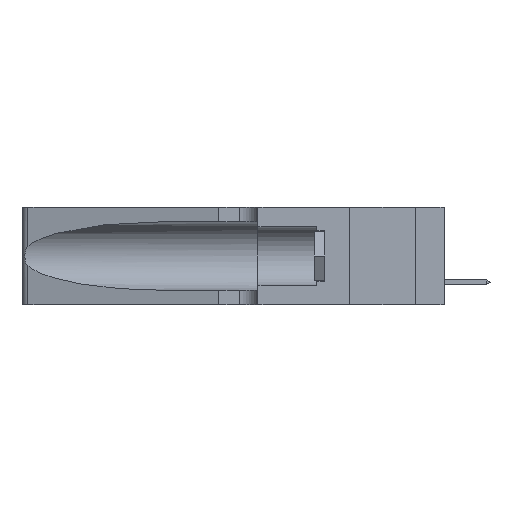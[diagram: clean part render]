
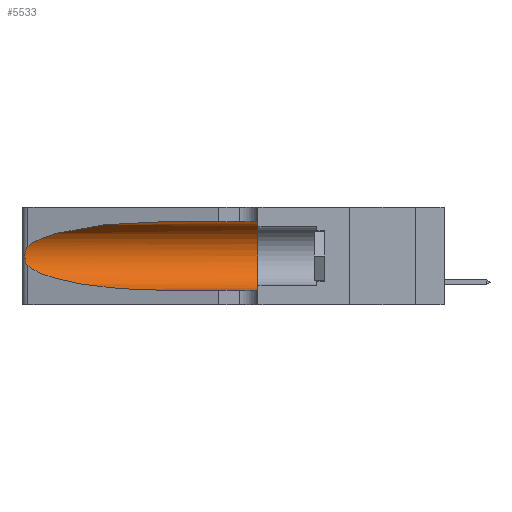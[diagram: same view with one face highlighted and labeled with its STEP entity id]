
A CAD part, left-side view. The second image highlights one B-rep face of the part: STEP entity #5533.
In plain terms, the highlighted cylindrical face has radius 3.308 mm (diameter 6.617 mm), a partial arc.
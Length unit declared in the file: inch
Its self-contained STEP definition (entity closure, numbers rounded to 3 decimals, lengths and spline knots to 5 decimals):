
#84 = CARTESIAN_POINT ( 'NONE',  ( 0.1305, 1.61858, 0.31525 ) ) ;
#409 = CARTESIAN_POINT ( 'NONE',  ( 0.1305, 0.72297, 0.05475 ) ) ;
#952 = CARTESIAN_POINT ( 'NONE',  ( 0.25487, 1.22718, 0.22369 ) ) ;
#1213 = EDGE_LOOP ( 'NONE', ( #17877, #12531, #1446, #14949, #14070, #15062 ) ) ;
#1439 = CARTESIAN_POINT ( 'NONE',  ( 0.25487, 1.22718, 0.14631 ) ) ;
#1446 = ORIENTED_EDGE ( 'NONE', *, *, #3852, .T. ) ;
#1830 = CARTESIAN_POINT ( 'NONE',  ( 0.1305, 1.61858, 0.05475 ) ) ;
#2104 =( BOUNDED_CURVE ( )  B_SPLINE_CURVE ( 3, ( #17723, #7977, #3104, #14460 ),
 .UNSPECIFIED., .F., .F. ) 
 B_SPLINE_CURVE_WITH_KNOTS ( ( 4, 4 ),
 ( 1.5708, 2.84003 ),
 .UNSPECIFIED. ) 
 CURVE ( )  GEOMETRIC_REPRESENTATION_ITEM ( )  RATIONAL_B_SPLINE_CURVE ( ( 1., 0.87, 0.87, 1. ) ) 
 REPRESENTATION_ITEM ( '' )  );
#3032 =( BOUNDED_CURVE ( )  B_SPLINE_CURVE ( 3, ( #16260, #19619, #20978, #14747 ),
 .UNSPECIFIED., .F., .F. ) 
 B_SPLINE_CURVE_WITH_KNOTS ( ( 4, 4 ),
 ( 3.44316, 4.71239 ),
 .UNSPECIFIED. ) 
 CURVE ( )  GEOMETRIC_REPRESENTATION_ITEM ( )  RATIONAL_B_SPLINE_CURVE ( ( 1., 0.87, 0.87, 1. ) ) 
 REPRESENTATION_ITEM ( '' )  );
#3104 = CARTESIAN_POINT ( 'NONE',  ( 0.2373, 1.15595, 0.28018 ) ) ;
#3233 = CARTESIAN_POINT ( 'NONE',  ( 0.25487, 1.22718, 0.14631 ) ) ;
#3531 = CARTESIAN_POINT ( 'NONE',  ( 0.26075, 1.23896, 0.19203 ) ) ;
#3852 = EDGE_CURVE ( 'NONE', #15073, #16967, #3032, .T. ) ;
#4428 = VECTOR ( 'NONE', #20040, 39.37008 ) ;
#5533 = ADVANCED_FACE ( 'NONE', ( #15386 ), #6993, .F. ) ;
#5790 = CIRCLE ( 'NONE', #17038, 0.13025 ) ;
#6338 = DIRECTION ( 'NONE',  ( 0., 1., 0. ) ) ;
#6527 = EDGE_CURVE ( 'NONE', #20601, #10795, #18376, .T. ) ;
#6926 = CARTESIAN_POINT ( 'NONE',  ( 0.1305, 0.72297, 0.31525 ) ) ;
#6978 = CARTESIAN_POINT ( 'NONE',  ( 0.25639, 1.23184, 0.21858 ) ) ;
#6993 = CYLINDRICAL_SURFACE ( 'NONE', #17171, 0.13025 ) ;
#7679 = VECTOR ( 'NONE', #14962, 39.37008 ) ;
#7977 = CARTESIAN_POINT ( 'NONE',  ( 0.18966, 0.96281, 0.31525 ) ) ;
#8276 = CARTESIAN_POINT ( 'NONE',  ( 0.25856, 1.23593, 0.16098 ) ) ;
#10487 = CARTESIAN_POINT ( 'NONE',  ( 0.1305, 1.61858, 0.185 ) ) ;
#10498 = LINE ( 'NONE', #1830, #7679 ) ;
#10795 = VERTEX_POINT ( 'NONE', #16656 ) ;
#11136 = DIRECTION ( 'NONE',  ( 0., 0., 1. ) ) ;
#11383 = CARTESIAN_POINT ( 'NONE',  ( 0.25555, 1.22994, 0.2215 ) ) ;
#12531 = ORIENTED_EDGE ( 'NONE', *, *, #17068, .T. ) ;
#12681 = CARTESIAN_POINT ( 'NONE',  ( 0.26017, 1.23833, 0.17102 ) ) ;
#13431 = CARTESIAN_POINT ( 'NONE',  ( 0.25555, 1.22993, 0.14849 ) ) ;
#13595 = DIRECTION ( 'NONE',  ( 0., -1., 0. ) ) ;
#14036 = EDGE_CURVE ( 'NONE', #20601, #18827, #2104, .T. ) ;
#14070 = ORIENTED_EDGE ( 'NONE', *, *, #16596, .F. ) ;
#14181 = CARTESIAN_POINT ( 'NONE',  ( 0.1305, 0.35, 0.05475 ) ) ;
#14424 = CARTESIAN_POINT ( 'NONE',  ( 0.25487, 1.22718, 0.22369 ) ) ;
#14460 = CARTESIAN_POINT ( 'NONE',  ( 0.25487, 1.22718, 0.22369 ) ) ;
#14747 = CARTESIAN_POINT ( 'NONE',  ( 0.1305, 0.72297, 0.05475 ) ) ;
#14949 = ORIENTED_EDGE ( 'NONE', *, *, #18521, .T. ) ;
#14962 = DIRECTION ( 'NONE',  ( 0., -1., 0. ) ) ;
#14972 = CARTESIAN_POINT ( 'NONE',  ( 0.26075, 1.23896, 0.178 ) ) ;
#15062 = ORIENTED_EDGE ( 'NONE', *, *, #6527, .F. ) ;
#15073 = VERTEX_POINT ( 'NONE', #3233 ) ;
#15386 = FACE_OUTER_BOUND ( 'NONE', #1213, .T. ) ;
#16260 = CARTESIAN_POINT ( 'NONE',  ( 0.25487, 1.22718, 0.14631 ) ) ;
#16596 = EDGE_CURVE ( 'NONE', #10795, #18245, #5790, .T. ) ;
#16656 = CARTESIAN_POINT ( 'NONE',  ( 0.1305, 0.35, 0.31525 ) ) ;
#16800 = CARTESIAN_POINT ( 'NONE',  ( 0.26018, 1.23835, 0.19895 ) ) ;
#16967 = VERTEX_POINT ( 'NONE', #409 ) ;
#17038 = AXIS2_PLACEMENT_3D ( 'NONE', #19441, #6338, #11136 ) ;
#17068 = EDGE_CURVE ( 'NONE', #18827, #15073, #17843, .T. ) ;
#17171 = AXIS2_PLACEMENT_3D ( 'NONE', #10487, #13595, #18428 ) ;
#17615 = CARTESIAN_POINT ( 'NONE',  ( 0.25639, 1.23186, 0.15144 ) ) ;
#17723 = CARTESIAN_POINT ( 'NONE',  ( 0.1305, 0.72297, 0.31525 ) ) ;
#17843 = B_SPLINE_CURVE_WITH_KNOTS ( 'NONE', 3,
 ( #14424, #11383, #6978, #20900, #20437, #16800, #3531, #14972, #12681, #8276, #19789, #17615, #13431, #1439 ),
 .UNSPECIFIED., .F., .F.,
 ( 4, 2, 2, 2, 2, 2, 4 ),
 ( 0., 0.00027, 0.00053, 0.00107, 0.0016, 0.00187, 0.00214 ),
 .UNSPECIFIED. ) ;
#17877 = ORIENTED_EDGE ( 'NONE', *, *, #14036, .T. ) ;
#18245 = VERTEX_POINT ( 'NONE', #14181 ) ;
#18376 = LINE ( 'NONE', #84, #4428 ) ;
#18428 = DIRECTION ( 'NONE',  ( 0., 0., -1. ) ) ;
#18521 = EDGE_CURVE ( 'NONE', #16967, #18245, #10498, .T. ) ;
#18827 = VERTEX_POINT ( 'NONE', #952 ) ;
#19441 = CARTESIAN_POINT ( 'NONE',  ( 0.1305, 0.35, 0.185 ) ) ;
#19619 = CARTESIAN_POINT ( 'NONE',  ( 0.2373, 1.15595, 0.08982 ) ) ;
#19789 = CARTESIAN_POINT ( 'NONE',  ( 0.25789, 1.23486, 0.15765 ) ) ;
#20040 = DIRECTION ( 'NONE',  ( 0., -1., 0. ) ) ;
#20437 = CARTESIAN_POINT ( 'NONE',  ( 0.25854, 1.2359, 0.20912 ) ) ;
#20601 = VERTEX_POINT ( 'NONE', #6926 ) ;
#20900 = CARTESIAN_POINT ( 'NONE',  ( 0.25787, 1.23484, 0.2124 ) ) ;
#20978 = CARTESIAN_POINT ( 'NONE',  ( 0.18966, 0.96281, 0.05475 ) ) ;
